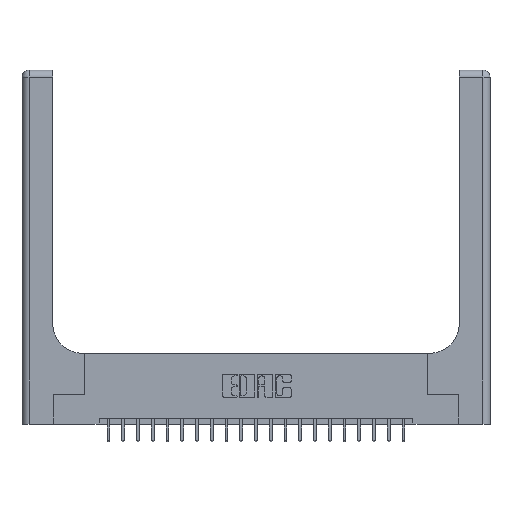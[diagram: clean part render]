
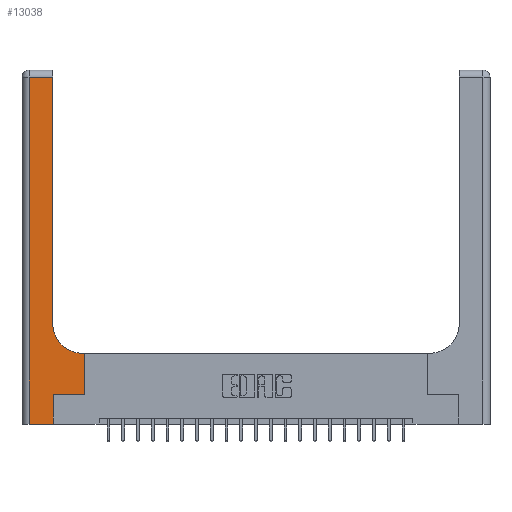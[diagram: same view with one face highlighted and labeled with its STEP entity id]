
A CAD part, top view. The second image highlights one B-rep face of the part: STEP entity #13038.
In plain terms, the highlighted planar face has unit normal (0, 0, 1).
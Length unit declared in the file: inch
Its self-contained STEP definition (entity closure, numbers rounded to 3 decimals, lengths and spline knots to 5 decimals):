
#958 = LINE ( 'NONE', #4861, #13450 ) ;
#1314 = EDGE_LOOP ( 'NONE', ( #10451, #7221, #21555, #13342, #20519, #18385, #9722, #20314, #4110 ) ) ;
#1847 = VERTEX_POINT ( 'NONE', #17057 ) ;
#1911 = AXIS2_PLACEMENT_3D ( 'NONE', #18199, #16176, #19668 ) ;
#2284 = LINE ( 'NONE', #12617, #4400 ) ;
#2295 = CARTESIAN_POINT ( 'NONE',  ( 0.06, 0., 0.37 ) ) ;
#3097 = CARTESIAN_POINT ( 'NONE',  ( 0.06, 3., 0.37 ) ) ;
#3257 = CARTESIAN_POINT ( 'NONE',  ( 0.265, 0.25, 0.37 ) ) ;
#3983 = EDGE_CURVE ( 'NONE', #8127, #14601, #8489, .T. ) ;
#4110 = ORIENTED_EDGE ( 'NONE', *, *, #18797, .T. ) ;
#4400 = VECTOR ( 'NONE', #14508, 39.37008 ) ;
#4446 = CARTESIAN_POINT ( 'NONE',  ( 0., 0., 0.37 ) ) ;
#4861 = CARTESIAN_POINT ( 'NONE',  ( 0.26, 0.6, 0.37 ) ) ;
#4968 = CARTESIAN_POINT ( 'NONE',  ( 0., 2.94, 0.37 ) ) ;
#5222 = EDGE_CURVE ( 'NONE', #14791, #11340, #958, .T. ) ;
#5422 = DIRECTION ( 'NONE',  ( 0., 1., 0. ) ) ;
#6429 = DIRECTION ( 'NONE',  ( 0., 1., 0. ) ) ;
#6621 = CARTESIAN_POINT ( 'NONE',  ( 0.265, 0., 0.37 ) ) ;
#7221 = ORIENTED_EDGE ( 'NONE', *, *, #18971, .T. ) ;
#7817 = DIRECTION ( 'NONE',  ( -1., 0., 0. ) ) ;
#8127 = VERTEX_POINT ( 'NONE', #18318 ) ;
#8375 = DIRECTION ( 'NONE',  ( 0., 0., -1. ) ) ;
#8382 = CIRCLE ( 'NONE', #1911, 0.25 ) ;
#8489 = LINE ( 'NONE', #3097, #18764 ) ;
#8675 = LINE ( 'NONE', #15500, #9737 ) ;
#9722 = ORIENTED_EDGE ( 'NONE', *, *, #20253, .T. ) ;
#9737 = VECTOR ( 'NONE', #5422, 39.37008 ) ;
#9939 = PLANE ( 'NONE',  #15390 ) ;
#10451 = ORIENTED_EDGE ( 'NONE', *, *, #15212, .T. ) ;
#10712 = CARTESIAN_POINT ( 'NONE',  ( 0.528, 0.6, 0.37 ) ) ;
#11239 = VECTOR ( 'NONE', #12701, 39.37008 ) ;
#11340 = VERTEX_POINT ( 'NONE', #14324 ) ;
#11386 = LINE ( 'NONE', #4446, #18795 ) ;
#11618 = CARTESIAN_POINT ( 'NONE',  ( 0., 3., 0.37 ) ) ;
#11642 = VECTOR ( 'NONE', #6429, 39.37008 ) ;
#11794 = DIRECTION ( 'NONE',  ( -1., 0., 0. ) ) ;
#12617 = CARTESIAN_POINT ( 'NONE',  ( 0.265, 0.25, 0.37 ) ) ;
#12701 = DIRECTION ( 'NONE',  ( 0., 1., 0. ) ) ;
#13038 = ADVANCED_FACE ( 'NONE', ( #13203 ), #9939, .F. ) ;
#13051 = CARTESIAN_POINT ( 'NONE',  ( 0.265, 0., 0.37 ) ) ;
#13203 = FACE_OUTER_BOUND ( 'NONE', #1314, .T. ) ;
#13342 = ORIENTED_EDGE ( 'NONE', *, *, #19669, .T. ) ;
#13450 = VECTOR ( 'NONE', #7817, 39.37008 ) ;
#14324 = CARTESIAN_POINT ( 'NONE',  ( 0.51, 0.6, 0.37 ) ) ;
#14508 = DIRECTION ( 'NONE',  ( 1., 0., 0. ) ) ;
#14597 = CARTESIAN_POINT ( 'NONE',  ( 0.26, 0.85, 0.37 ) ) ;
#14601 = VERTEX_POINT ( 'NONE', #2295 ) ;
#14791 = VERTEX_POINT ( 'NONE', #10712 ) ;
#14845 = DIRECTION ( 'NONE',  ( 1., 0., 0. ) ) ;
#15143 = LINE ( 'NONE', #4968, #15887 ) ;
#15212 = EDGE_CURVE ( 'NONE', #18735, #1847, #8675, .T. ) ;
#15390 = AXIS2_PLACEMENT_3D ( 'NONE', #11618, #8375, #18464 ) ;
#15500 = CARTESIAN_POINT ( 'NONE',  ( 0.26, 3., 0.37 ) ) ;
#15663 = VERTEX_POINT ( 'NONE', #16263 ) ;
#15887 = VECTOR ( 'NONE', #11794, 39.37008 ) ;
#16176 = DIRECTION ( 'NONE',  ( 0., 0., -1. ) ) ;
#16263 = CARTESIAN_POINT ( 'NONE',  ( 0.528, 0.25, 0.37 ) ) ;
#17026 = VERTEX_POINT ( 'NONE', #6621 ) ;
#17057 = CARTESIAN_POINT ( 'NONE',  ( 0.26, 2.94, 0.37 ) ) ;
#17272 = EDGE_CURVE ( 'NONE', #17392, #15663, #2284, .T. ) ;
#17392 = VERTEX_POINT ( 'NONE', #3257 ) ;
#18199 = CARTESIAN_POINT ( 'NONE',  ( 0.51, 0.85, 0.37 ) ) ;
#18318 = CARTESIAN_POINT ( 'NONE',  ( 0.06, 2.94, 0.37 ) ) ;
#18385 = ORIENTED_EDGE ( 'NONE', *, *, #17272, .T. ) ;
#18464 = DIRECTION ( 'NONE',  ( -1., 0., 0. ) ) ;
#18586 = DIRECTION ( 'NONE',  ( 0., -1., 0. ) ) ;
#18735 = VERTEX_POINT ( 'NONE', #14597 ) ;
#18764 = VECTOR ( 'NONE', #18586, 39.37008 ) ;
#18795 = VECTOR ( 'NONE', #14845, 39.37008 ) ;
#18797 = EDGE_CURVE ( 'NONE', #11340, #18735, #8382, .T. ) ;
#18842 = EDGE_CURVE ( 'NONE', #17026, #17392, #21569, .T. ) ;
#18971 = EDGE_CURVE ( 'NONE', #1847, #8127, #15143, .T. ) ;
#19668 = DIRECTION ( 'NONE',  ( 1., 0., 0. ) ) ;
#19669 = EDGE_CURVE ( 'NONE', #14601, #17026, #11386, .T. ) ;
#20253 = EDGE_CURVE ( 'NONE', #15663, #14791, #22127, .T. ) ;
#20314 = ORIENTED_EDGE ( 'NONE', *, *, #5222, .T. ) ;
#20437 = CARTESIAN_POINT ( 'NONE',  ( 0.528, 0.25, 0.37 ) ) ;
#20519 = ORIENTED_EDGE ( 'NONE', *, *, #18842, .T. ) ;
#21555 = ORIENTED_EDGE ( 'NONE', *, *, #3983, .T. ) ;
#21569 = LINE ( 'NONE', #13051, #11239 ) ;
#22127 = LINE ( 'NONE', #20437, #11642 ) ;
